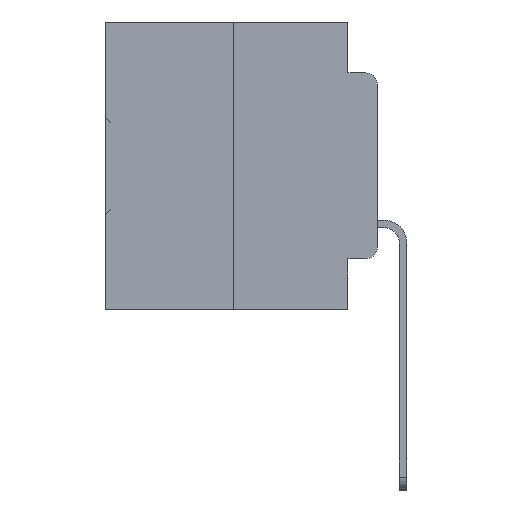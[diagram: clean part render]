
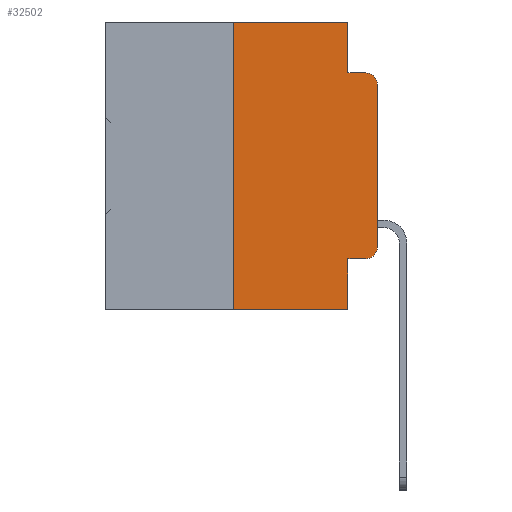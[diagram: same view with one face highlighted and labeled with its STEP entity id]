
A CAD part, left-side view. The second image highlights one B-rep face of the part: STEP entity #32502.
In plain terms, the highlighted planar face has unit normal (-1, 0, 0).
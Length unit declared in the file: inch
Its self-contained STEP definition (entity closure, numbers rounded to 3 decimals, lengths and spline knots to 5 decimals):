
#284 = LINE ( 'NONE', #20812, #21008 ) ;
#350 = VECTOR ( 'NONE', #5243, 39.37008 ) ;
#660 = VERTEX_POINT ( 'NONE', #24899 ) ;
#1234 = CARTESIAN_POINT ( 'NONE',  ( 0., 0.051, -0.4115 ) ) ;
#1400 = DIRECTION ( 'NONE',  ( 0., 0., -1. ) ) ;
#1567 = CARTESIAN_POINT ( 'NONE',  ( 0., 0.051, -0.0885 ) ) ;
#1763 = EDGE_CURVE ( 'NONE', #37512, #3704, #5459, .T. ) ;
#2219 = ORIENTED_EDGE ( 'NONE', *, *, #27881, .T. ) ;
#3566 = ORIENTED_EDGE ( 'NONE', *, *, #1763, .F. ) ;
#3704 = VERTEX_POINT ( 'NONE', #11900 ) ;
#3778 = EDGE_CURVE ( 'NONE', #6895, #37512, #35864, .T. ) ;
#4182 = ORIENTED_EDGE ( 'NONE', *, *, #27375, .T. ) ;
#4994 = ORIENTED_EDGE ( 'NONE', *, *, #31950, .T. ) ;
#5243 = DIRECTION ( 'NONE',  ( 0., -1., 0. ) ) ;
#5459 = LINE ( 'NONE', #25937, #21078 ) ;
#5809 = VERTEX_POINT ( 'NONE', #11927 ) ;
#5999 = VECTOR ( 'NONE', #1400, 39.37008 ) ;
#6895 = VERTEX_POINT ( 'NONE', #16826 ) ;
#6938 = VERTEX_POINT ( 'NONE', #37230 ) ;
#7467 = ORIENTED_EDGE ( 'NONE', *, *, #16684, .T. ) ;
#8416 = DIRECTION ( 'NONE',  ( 0., -1., 0. ) ) ;
#8840 = EDGE_CURVE ( 'NONE', #5809, #6895, #22807, .T. ) ;
#9286 = ORIENTED_EDGE ( 'NONE', *, *, #15649, .F. ) ;
#9302 = DIRECTION ( 'NONE',  ( 0., 0., -1. ) ) ;
#9852 = CARTESIAN_POINT ( 'NONE',  ( 0., 0., -0.3915 ) ) ;
#9898 = CARTESIAN_POINT ( 'NONE',  ( 0., 0.473, 0. ) ) ;
#10373 = VERTEX_POINT ( 'NONE', #1234 ) ;
#11447 = CARTESIAN_POINT ( 'NONE',  ( 0., 0.473, 0. ) ) ;
#11900 = CARTESIAN_POINT ( 'NONE',  ( 0., 0.02, -0.0885 ) ) ;
#11927 = CARTESIAN_POINT ( 'NONE',  ( 0., 0.25, 0. ) ) ;
#12134 = VECTOR ( 'NONE', #35682, 39.37008 ) ;
#12145 = CARTESIAN_POINT ( 'NONE',  ( 0., 0.051, 0. ) ) ;
#12844 = DIRECTION ( 'NONE',  ( 0., 0., -1. ) ) ;
#13050 = LINE ( 'NONE', #27108, #12134 ) ;
#13698 = EDGE_CURVE ( 'NONE', #6938, #5809, #13050, .T. ) ;
#14276 = AXIS2_PLACEMENT_3D ( 'NONE', #32814, #15442, #35745 ) ;
#14676 = AXIS2_PLACEMENT_3D ( 'NONE', #17579, #37878, #20521 ) ;
#14956 = DIRECTION ( 'NONE',  ( 0., -1., 0. ) ) ;
#15047 = VECTOR ( 'NONE', #26013, 39.37008 ) ;
#15442 = DIRECTION ( 'NONE',  ( -1., 0., 0. ) ) ;
#15649 = EDGE_CURVE ( 'NONE', #10373, #660, #31135, .T. ) ;
#15906 = VECTOR ( 'NONE', #36236, 39.37008 ) ;
#16297 = CARTESIAN_POINT ( 'NONE',  ( 0., 0., -0.1085 ) ) ;
#16684 = EDGE_CURVE ( 'NONE', #6938, #660, #31499, .T. ) ;
#16826 = CARTESIAN_POINT ( 'NONE',  ( 0., 0.051, 0. ) ) ;
#17579 = CARTESIAN_POINT ( 'NONE',  ( 0., 0.02, -0.3915 ) ) ;
#17644 = VERTEX_POINT ( 'NONE', #9852 ) ;
#18321 = EDGE_CURVE ( 'NONE', #17644, #29957, #31355, .T. ) ;
#20354 = ORIENTED_EDGE ( 'NONE', *, *, #18321, .T. ) ;
#20521 = DIRECTION ( 'NONE',  ( 0., 0., -1. ) ) ;
#20812 = CARTESIAN_POINT ( 'NONE',  ( 0., 0.051, -0.4115 ) ) ;
#21008 = VECTOR ( 'NONE', #14956, 39.37008 ) ;
#21078 = VECTOR ( 'NONE', #8416, 39.37008 ) ;
#21152 = AXIS2_PLACEMENT_3D ( 'NONE', #9898, #30275, #12844 ) ;
#22461 = ORIENTED_EDGE ( 'NONE', *, *, #13698, .F. ) ;
#22807 = LINE ( 'NONE', #11447, #15047 ) ;
#22905 = ORIENTED_EDGE ( 'NONE', *, *, #8840, .F. ) ;
#24613 = FACE_OUTER_BOUND ( 'NONE', #35883, .T. ) ;
#24899 = CARTESIAN_POINT ( 'NONE',  ( 0., 0.051, -0.5 ) ) ;
#24951 = CARTESIAN_POINT ( 'NONE',  ( 0., 0.051, 0. ) ) ;
#25937 = CARTESIAN_POINT ( 'NONE',  ( 0., 0.051, -0.0885 ) ) ;
#26013 = DIRECTION ( 'NONE',  ( 0., -1., 0. ) ) ;
#26229 = ORIENTED_EDGE ( 'NONE', *, *, #3778, .F. ) ;
#26292 = CARTESIAN_POINT ( 'NONE',  ( 0., 0.02, -0.4115 ) ) ;
#27108 = CARTESIAN_POINT ( 'NONE',  ( 0., 0.25, 0. ) ) ;
#27375 = EDGE_CURVE ( 'NONE', #10373, #33425, #284, .T. ) ;
#27393 = PLANE ( 'NONE',  #21152 ) ;
#27881 = EDGE_CURVE ( 'NONE', #33425, #17644, #34554, .T. ) ;
#28558 = CARTESIAN_POINT ( 'NONE',  ( 0., 0.473, -0.5 ) ) ;
#29957 = VERTEX_POINT ( 'NONE', #16297 ) ;
#30275 = DIRECTION ( 'NONE',  ( 1., 0., 0. ) ) ;
#30431 = CARTESIAN_POINT ( 'NONE',  ( 0., 0., 0. ) ) ;
#31135 = LINE ( 'NONE', #24951, #5999 ) ;
#31355 = LINE ( 'NONE', #30431, #15906 ) ;
#31499 = LINE ( 'NONE', #28558, #350 ) ;
#31950 = EDGE_CURVE ( 'NONE', #29957, #3704, #36847, .T. ) ;
#32502 = ADVANCED_FACE ( 'NONE', ( #24613 ), #27393, .F. ) ;
#32814 = CARTESIAN_POINT ( 'NONE',  ( 0., 0.02, -0.1085 ) ) ;
#33425 = VERTEX_POINT ( 'NONE', #26292 ) ;
#34554 = CIRCLE ( 'NONE', #14676, 0.02 ) ;
#34961 = VECTOR ( 'NONE', #9302, 39.37008 ) ;
#35682 = DIRECTION ( 'NONE',  ( 0., 0., 1. ) ) ;
#35745 = DIRECTION ( 'NONE',  ( 0., 0., -1. ) ) ;
#35864 = LINE ( 'NONE', #12145, #34961 ) ;
#35883 = EDGE_LOOP ( 'NONE', ( #20354, #4994, #3566, #26229, #22905, #22461, #7467, #9286, #4182, #2219 ) ) ;
#36236 = DIRECTION ( 'NONE',  ( 0., 0., 1. ) ) ;
#36847 = CIRCLE ( 'NONE', #14276, 0.02 ) ;
#37230 = CARTESIAN_POINT ( 'NONE',  ( 0., 0.25, -0.5 ) ) ;
#37512 = VERTEX_POINT ( 'NONE', #1567 ) ;
#37878 = DIRECTION ( 'NONE',  ( -1., 0., 0. ) ) ;
